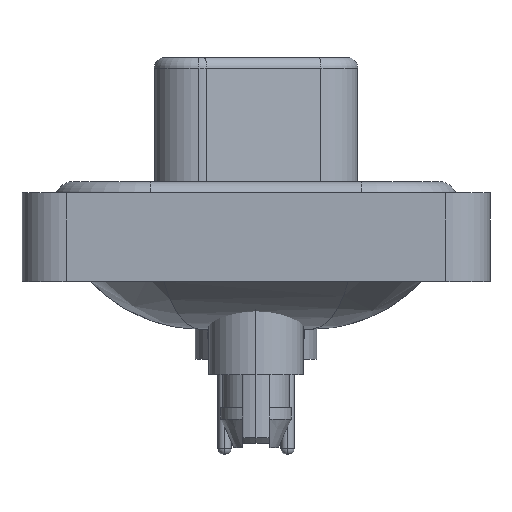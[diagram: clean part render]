
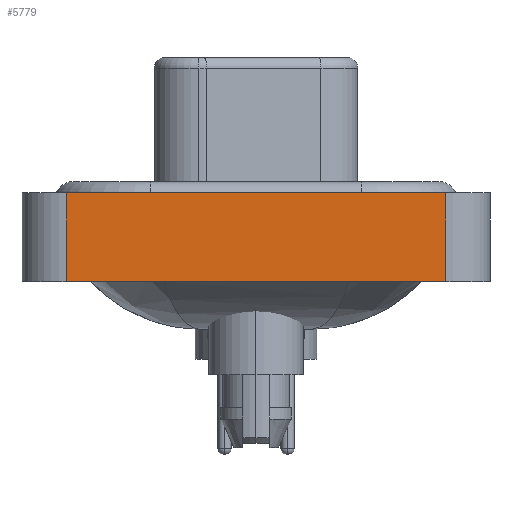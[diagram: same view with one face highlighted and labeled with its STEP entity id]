
A CAD part, left-side view. The second image highlights one B-rep face of the part: STEP entity #5779.
In plain terms, the highlighted planar face has unit normal (-1, 0, 0).
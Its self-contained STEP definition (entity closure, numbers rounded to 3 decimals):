
#380 = EDGE_CURVE ( 'NONE', #19655, #19978, #10006, .T. ) ;
#887 = CARTESIAN_POINT ( 'NONE',  ( -7.25, 8.55, -3.6 ) ) ;
#2352 = PLANE ( 'NONE',  #9548 ) ;
#3322 = DIRECTION ( 'NONE',  ( 0., -1., 0. ) ) ;
#3412 = VECTOR ( 'NONE', #3763, 1000. ) ;
#3654 = LINE ( 'NONE', #10629, #3412 ) ;
#3763 = DIRECTION ( 'NONE',  ( 0., 0., 1. ) ) ;
#5079 = CARTESIAN_POINT ( 'NONE',  ( -7.25, 8.55, 0.4 ) ) ;
#5336 = VECTOR ( 'NONE', #6559, 1000. ) ;
#5364 = LINE ( 'NONE', #20818, #14435 ) ;
#5779 = ADVANCED_FACE ( 'NONE', ( #9320 ), #2352, .T. ) ;
#6559 = DIRECTION ( 'NONE',  ( 0., -1., 0. ) ) ;
#7247 = VERTEX_POINT ( 'NONE', #887 ) ;
#7346 = ORIENTED_EDGE ( 'NONE', *, *, #16307, .T. ) ;
#9320 = FACE_OUTER_BOUND ( 'NONE', #12853, .T. ) ;
#9548 = AXIS2_PLACEMENT_3D ( 'NONE', #12884, #17669, #19827 ) ;
#10006 = LINE ( 'NONE', #15266, #5336 ) ;
#10309 = VECTOR ( 'NONE', #11626, 1000. ) ;
#10629 = CARTESIAN_POINT ( 'NONE',  ( -7.25, -8.55, -3.6 ) ) ;
#11626 = DIRECTION ( 'NONE',  ( 0., 0., 1. ) ) ;
#12853 = EDGE_LOOP ( 'NONE', ( #15191, #14534, #18075, #7346 ) ) ;
#12884 = CARTESIAN_POINT ( 'NONE',  ( -7.25, -8.55, -3.6 ) ) ;
#13119 = CARTESIAN_POINT ( 'NONE',  ( -7.25, -8.55, -3.6 ) ) ;
#13448 = LINE ( 'NONE', #20404, #10309 ) ;
#13670 = EDGE_CURVE ( 'NONE', #20499, #19978, #3654, .T. ) ;
#14435 = VECTOR ( 'NONE', #3322, 1000. ) ;
#14534 = ORIENTED_EDGE ( 'NONE', *, *, #380, .F. ) ;
#15191 = ORIENTED_EDGE ( 'NONE', *, *, #13670, .T. ) ;
#15266 = CARTESIAN_POINT ( 'NONE',  ( -7.25, -8.55, 0.4 ) ) ;
#16307 = EDGE_CURVE ( 'NONE', #7247, #20499, #5364, .T. ) ;
#17669 = DIRECTION ( 'NONE',  ( -1., 0., 0. ) ) ;
#18075 = ORIENTED_EDGE ( 'NONE', *, *, #20655, .F. ) ;
#19655 = VERTEX_POINT ( 'NONE', #5079 ) ;
#19827 = DIRECTION ( 'NONE',  ( 0., 0., 1. ) ) ;
#19978 = VERTEX_POINT ( 'NONE', #21487 ) ;
#20404 = CARTESIAN_POINT ( 'NONE',  ( -7.25, 8.55, -3.6 ) ) ;
#20499 = VERTEX_POINT ( 'NONE', #13119 ) ;
#20655 = EDGE_CURVE ( 'NONE', #7247, #19655, #13448, .T. ) ;
#20818 = CARTESIAN_POINT ( 'NONE',  ( -7.25, -8.55, -3.6 ) ) ;
#21487 = CARTESIAN_POINT ( 'NONE',  ( -7.25, -8.55, 0.4 ) ) ;
